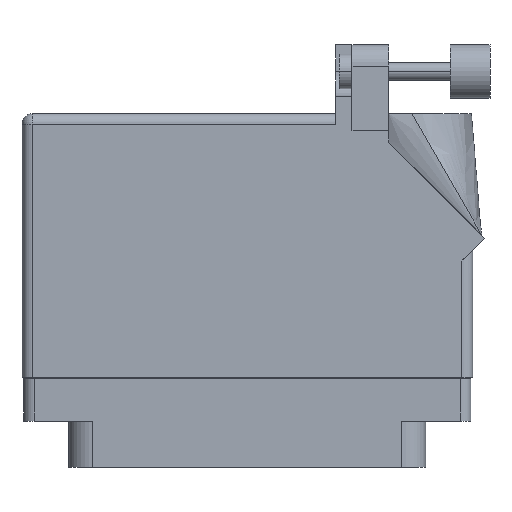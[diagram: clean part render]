
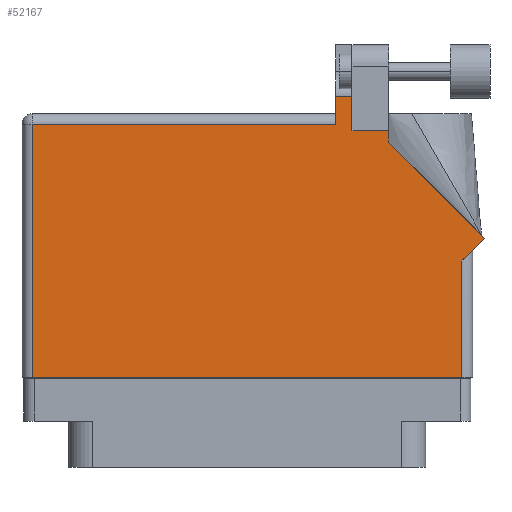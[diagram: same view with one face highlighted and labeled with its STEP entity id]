
A CAD part, front view. The second image highlights one B-rep face of the part: STEP entity #52167.
In plain terms, the highlighted face is planar.
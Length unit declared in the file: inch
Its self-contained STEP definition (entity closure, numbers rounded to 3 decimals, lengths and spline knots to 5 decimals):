
#15 = EDGE_CURVE ( 'NONE', #37387, #44317, #29954, .T. ) ;
#198 = CARTESIAN_POINT ( 'NONE',  ( 0.607, 1.33, 0.455 ) ) ;
#566 = VECTOR ( 'NONE', #24380, 39.37008 ) ;
#1108 = LINE ( 'NONE', #31077, #30156 ) ;
#2257 = DIRECTION ( 'NONE',  ( -1., 0., 0. ) ) ;
#2299 = ORIENTED_EDGE ( 'NONE', *, *, #28271, .T. ) ;
#2448 = ORIENTED_EDGE ( 'NONE', *, *, #3124, .T. ) ;
#3038 = DIRECTION ( 'NONE',  ( 0., -1., 0. ) ) ;
#3124 = EDGE_CURVE ( 'NONE', #33677, #47149, #18264, .T. ) ;
#5166 = CARTESIAN_POINT ( 'NONE',  ( 1.244, 0.637, 0.455 ) ) ;
#5530 = CARTESIAN_POINT ( 'NONE',  ( 0.513, 1.368, 0.455 ) ) ;
#5599 = PLANE ( 'NONE',  #52244 ) ;
#6296 = LINE ( 'NONE', #17638, #23997 ) ;
#6766 = CARTESIAN_POINT ( 'NONE',  ( 0.513, 1.43, 0.455 ) ) ;
#6780 = CARTESIAN_POINT ( 'NONE',  ( 1.306, 0.637, 0.455 ) ) ;
#7592 = LINE ( 'NONE', #5166, #32973 ) ;
#7726 = DIRECTION ( 'NONE',  ( 1., 0., 0. ) ) ;
#7992 = VERTEX_POINT ( 'NONE', #10352 ) ;
#8420 = CARTESIAN_POINT ( 'NONE',  ( 0.82, 1.26442, 0.455 ) ) ;
#8940 = VECTOR ( 'NONE', #3038, 39.37008 ) ;
#9072 = EDGE_CURVE ( 'NONE', #47149, #29763, #49889, .T. ) ;
#9807 = EDGE_CURVE ( 'NONE', #21515, #44718, #12623, .T. ) ;
#9849 = ORIENTED_EDGE ( 'NONE', *, *, #9807, .T. ) ;
#9860 = CARTESIAN_POINT ( 'NONE',  ( 0.513, 1.5315, 0.455 ) ) ;
#10352 = CARTESIAN_POINT ( 'NONE',  ( 0.82, 1.26442, 0.455 ) ) ;
#11076 = CARTESIAN_POINT ( 'NONE',  ( 1.244, -0.1, 0.455 ) ) ;
#12623 = LINE ( 'NONE', #24357, #28447 ) ;
#13789 = VERTEX_POINT ( 'NONE', #5530 ) ;
#14124 = VERTEX_POINT ( 'NONE', #48299 ) ;
#14656 = DIRECTION ( 'NONE',  ( -0.707, 0.707, 0. ) ) ;
#15698 = ORIENTED_EDGE ( 'NONE', *, *, #16241, .T. ) ;
#16241 = EDGE_CURVE ( 'NONE', #7992, #33677, #34949, .T. ) ;
#17194 = EDGE_CURVE ( 'NONE', #13789, #14124, #29086, .T. ) ;
#17638 = CARTESIAN_POINT ( 'NONE',  ( -1.244, -0.1, 0.455 ) ) ;
#18026 = VERTEX_POINT ( 'NONE', #9860 ) ;
#18144 = DIRECTION ( 'NONE',  ( 0., -1., 0. ) ) ;
#18264 = LINE ( 'NONE', #46510, #27750 ) ;
#20133 = CARTESIAN_POINT ( 'NONE',  ( -1.306, 1.368, 0.455 ) ) ;
#20277 = CARTESIAN_POINT ( 'NONE',  ( 1.37671, 0.70771, 0.455 ) ) ;
#20732 = CARTESIAN_POINT ( 'NONE',  ( -1.244, -0.1, 0.455 ) ) ;
#20760 = CARTESIAN_POINT ( 'NONE',  ( 0.607, 1.33, 0.455 ) ) ;
#21243 = DIRECTION ( 'NONE',  ( 0., 1., 0. ) ) ;
#21400 = LINE ( 'NONE', #40765, #566 ) ;
#21515 = VERTEX_POINT ( 'NONE', #20732 ) ;
#22416 = DIRECTION ( 'NONE',  ( -1., 0., 0. ) ) ;
#23410 = VECTOR ( 'NONE', #52018, 39.37008 ) ;
#23997 = VECTOR ( 'NONE', #18144, 39.37008 ) ;
#24357 = CARTESIAN_POINT ( 'NONE',  ( -1.306, -0.1, 0.455 ) ) ;
#24380 = DIRECTION ( 'NONE',  ( -1., 0., 0. ) ) ;
#25697 = ORIENTED_EDGE ( 'NONE', *, *, #49875, .T. ) ;
#26064 = EDGE_CURVE ( 'NONE', #44317, #7992, #1108, .T. ) ;
#27750 = VECTOR ( 'NONE', #2257, 39.37008 ) ;
#28271 = EDGE_CURVE ( 'NONE', #44718, #37387, #7592, .T. ) ;
#28447 = VECTOR ( 'NONE', #7726, 39.37008 ) ;
#28573 = ORIENTED_EDGE ( 'NONE', *, *, #42840, .T. ) ;
#29086 = LINE ( 'NONE', #20133, #23410 ) ;
#29763 = VERTEX_POINT ( 'NONE', #36188 ) ;
#29954 = LINE ( 'NONE', #6780, #50039 ) ;
#30156 = VECTOR ( 'NONE', #14656, 39.37008 ) ;
#30987 = ORIENTED_EDGE ( 'NONE', *, *, #9072, .T. ) ;
#31077 = CARTESIAN_POINT ( 'NONE',  ( 1.37671, 0.70771, 0.455 ) ) ;
#32296 = ORIENTED_EDGE ( 'NONE', *, *, #15, .T. ) ;
#32361 = VECTOR ( 'NONE', #36596, 39.37008 ) ;
#32973 = VECTOR ( 'NONE', #21243, 39.37008 ) ;
#33647 = ORIENTED_EDGE ( 'NONE', *, *, #17194, .T. ) ;
#33677 = VERTEX_POINT ( 'NONE', #45037 ) ;
#34226 = CARTESIAN_POINT ( 'NONE',  ( 1.244, 0.575, 0.455 ) ) ;
#34545 = FACE_OUTER_BOUND ( 'NONE', #46163, .T. ) ;
#34949 = LINE ( 'NONE', #8420, #49360 ) ;
#35199 = ORIENTED_EDGE ( 'NONE', *, *, #26064, .T. ) ;
#36188 = CARTESIAN_POINT ( 'NONE',  ( 0.607, 1.5315, 0.455 ) ) ;
#36596 = DIRECTION ( 'NONE',  ( 0., 1., 0. ) ) ;
#37387 = VERTEX_POINT ( 'NONE', #34226 ) ;
#40716 = DIRECTION ( 'NONE',  ( 0., 1., 0. ) ) ;
#40765 = CARTESIAN_POINT ( 'NONE',  ( 0.93777, 1.5315, 0.455 ) ) ;
#41138 = LINE ( 'NONE', #6766, #8940 ) ;
#42397 = ORIENTED_EDGE ( 'NONE', *, *, #43756, .T. ) ;
#42840 = EDGE_CURVE ( 'NONE', #18026, #13789, #41138, .T. ) ;
#43756 = EDGE_CURVE ( 'NONE', #14124, #21515, #6296, .T. ) ;
#44317 = VERTEX_POINT ( 'NONE', #20277 ) ;
#44718 = VERTEX_POINT ( 'NONE', #11076 ) ;
#45037 = CARTESIAN_POINT ( 'NONE',  ( 0.82, 1.33, 0.455 ) ) ;
#46163 = EDGE_LOOP ( 'NONE', ( #30987, #25697, #28573, #33647, #42397, #9849, #2299, #32296, #35199, #15698, #2448 ) ) ;
#46504 = CARTESIAN_POINT ( 'NONE',  ( -1.306, 1.43, 0.455 ) ) ;
#46510 = CARTESIAN_POINT ( 'NONE',  ( 0.82, 1.33, 0.455 ) ) ;
#46973 = DIRECTION ( 'NONE',  ( 0.707, 0.707, 0. ) ) ;
#47149 = VERTEX_POINT ( 'NONE', #20760 ) ;
#48299 = CARTESIAN_POINT ( 'NONE',  ( -1.244, 1.368, 0.455 ) ) ;
#49360 = VECTOR ( 'NONE', #40716, 39.37008 ) ;
#49875 = EDGE_CURVE ( 'NONE', #29763, #18026, #21400, .T. ) ;
#49889 = LINE ( 'NONE', #198, #32361 ) ;
#50039 = VECTOR ( 'NONE', #46973, 39.37008 ) ;
#50523 = DIRECTION ( 'NONE',  ( 0., 0., -1. ) ) ;
#52018 = DIRECTION ( 'NONE',  ( -1., 0., 0. ) ) ;
#52167 = ADVANCED_FACE ( 'NONE', ( #34545 ), #5599, .F. ) ;
#52244 = AXIS2_PLACEMENT_3D ( 'NONE', #46504, #50523, #22416 ) ;
